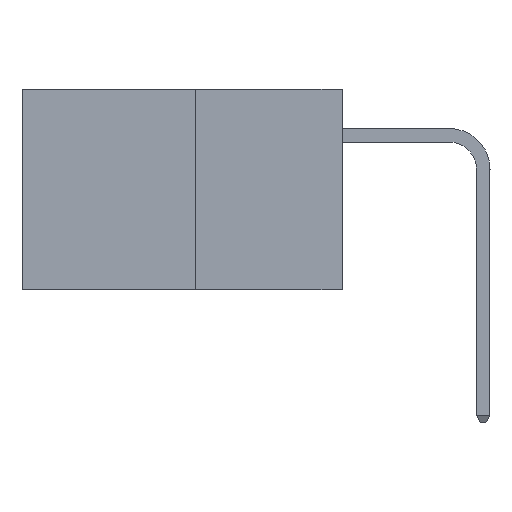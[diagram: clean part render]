
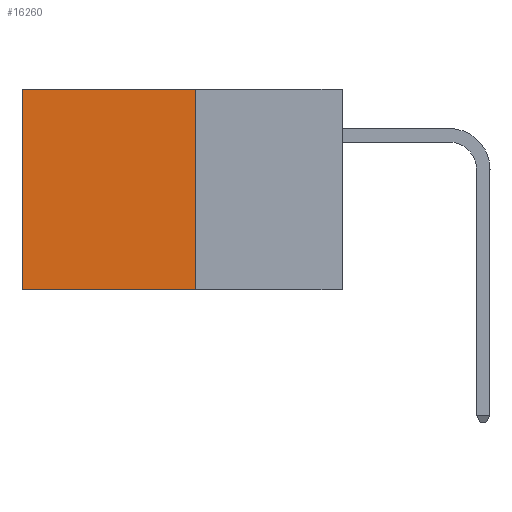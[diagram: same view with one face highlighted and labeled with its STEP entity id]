
A CAD part, left-side view. The second image highlights one B-rep face of the part: STEP entity #16260.
In plain terms, the highlighted planar face has unit normal (-1, 0, 0).
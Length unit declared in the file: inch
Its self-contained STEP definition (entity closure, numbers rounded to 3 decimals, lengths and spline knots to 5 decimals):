
#119 = LINE ( 'NONE', #2873, #13411 ) ;
#589 = VECTOR ( 'NONE', #17332, 39.37008 ) ;
#795 = VERTEX_POINT ( 'NONE', #20791 ) ;
#948 = LINE ( 'NONE', #6377, #5412 ) ;
#1351 = DIRECTION ( 'NONE',  ( 0., 1., 0. ) ) ;
#1735 = EDGE_LOOP ( 'NONE', ( #12289, #18108, #10492, #8138 ) ) ;
#2532 = VECTOR ( 'NONE', #6896, 39.37008 ) ;
#2873 = CARTESIAN_POINT ( 'NONE',  ( 0.277, 0.27, -0.37 ) ) ;
#3537 = EDGE_CURVE ( 'NONE', #795, #7203, #119, .T. ) ;
#4846 = VERTEX_POINT ( 'NONE', #8213 ) ;
#4855 = EDGE_CURVE ( 'NONE', #7203, #4846, #13357, .T. ) ;
#5412 = VECTOR ( 'NONE', #1351, 39.37008 ) ;
#6377 = CARTESIAN_POINT ( 'NONE',  ( 0.277, 0.27, 0. ) ) ;
#6896 = DIRECTION ( 'NONE',  ( 0., 0., -1. ) ) ;
#6982 = CARTESIAN_POINT ( 'NONE',  ( 0.277, 0.27, -0.37 ) ) ;
#7203 = VERTEX_POINT ( 'NONE', #6982 ) ;
#7425 = AXIS2_PLACEMENT_3D ( 'NONE', #7439, #9112, #20458 ) ;
#7439 = CARTESIAN_POINT ( 'NONE',  ( 0.277, 0.27, -0.37 ) ) ;
#8138 = ORIENTED_EDGE ( 'NONE', *, *, #18806, .T. ) ;
#8213 = CARTESIAN_POINT ( 'NONE',  ( 0.277, 0.59, -0.37 ) ) ;
#9112 = DIRECTION ( 'NONE',  ( 1., 0., 0. ) ) ;
#9281 = CARTESIAN_POINT ( 'NONE',  ( 0.277, 0.59, 0. ) ) ;
#10492 = ORIENTED_EDGE ( 'NONE', *, *, #3537, .F. ) ;
#10522 = FACE_OUTER_BOUND ( 'NONE', #1735, .T. ) ;
#12289 = ORIENTED_EDGE ( 'NONE', *, *, #18336, .T. ) ;
#13357 = LINE ( 'NONE', #17481, #589 ) ;
#13411 = VECTOR ( 'NONE', #17077, 39.37008 ) ;
#14472 = VERTEX_POINT ( 'NONE', #9281 ) ;
#15107 = CARTESIAN_POINT ( 'NONE',  ( 0.277, 0.59, -0.37 ) ) ;
#16260 = ADVANCED_FACE ( 'NONE', ( #10522 ), #17250, .F. ) ;
#16293 = LINE ( 'NONE', #15107, #2532 ) ;
#17077 = DIRECTION ( 'NONE',  ( 0., 0., -1. ) ) ;
#17250 = PLANE ( 'NONE',  #7425 ) ;
#17332 = DIRECTION ( 'NONE',  ( 0., 1., 0. ) ) ;
#17481 = CARTESIAN_POINT ( 'NONE',  ( 0.277, 0.27, -0.37 ) ) ;
#18108 = ORIENTED_EDGE ( 'NONE', *, *, #4855, .F. ) ;
#18336 = EDGE_CURVE ( 'NONE', #14472, #4846, #16293, .T. ) ;
#18806 = EDGE_CURVE ( 'NONE', #795, #14472, #948, .T. ) ;
#20458 = DIRECTION ( 'NONE',  ( 0., 0., -1. ) ) ;
#20791 = CARTESIAN_POINT ( 'NONE',  ( 0.277, 0.27, 0. ) ) ;
